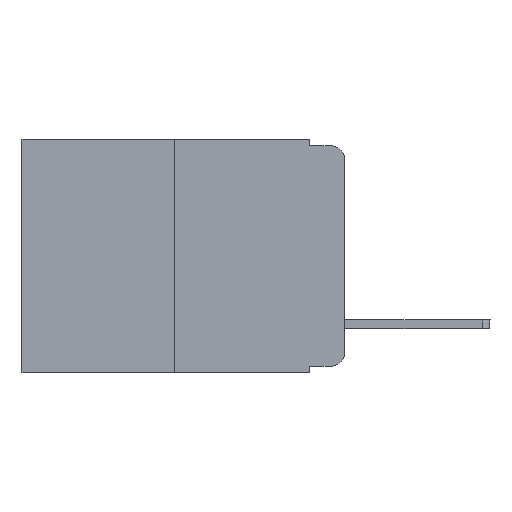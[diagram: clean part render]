
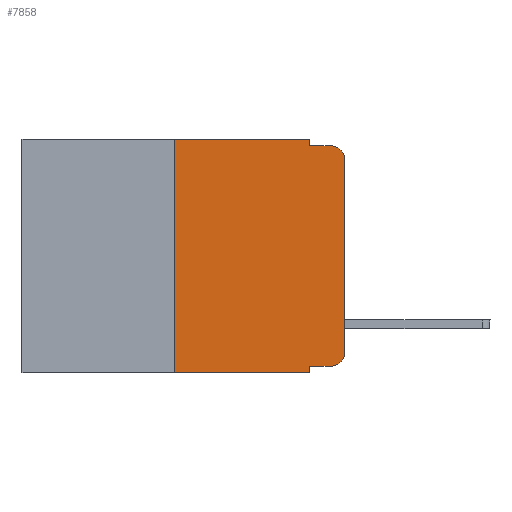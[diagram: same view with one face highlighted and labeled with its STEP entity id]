
A CAD part, left-side view. The second image highlights one B-rep face of the part: STEP entity #7858.
In plain terms, the highlighted planar face has unit normal (-1, 0, 0).
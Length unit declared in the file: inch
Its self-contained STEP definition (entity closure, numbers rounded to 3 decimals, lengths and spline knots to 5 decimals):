
#303 = DIRECTION ( 'NONE',  ( 0., 0., -1. ) ) ;
#461 = CARTESIAN_POINT ( 'NONE',  ( 0., 0., -0.03 ) ) ;
#546 = DIRECTION ( 'NONE',  ( 0., -1., 0. ) ) ;
#664 = VECTOR ( 'NONE', #1837, 39.37008 ) ;
#684 = ORIENTED_EDGE ( 'NONE', *, *, #11187, .F. ) ;
#804 = ORIENTED_EDGE ( 'NONE', *, *, #11009, .F. ) ;
#863 = LINE ( 'NONE', #10793, #5171 ) ;
#924 = DIRECTION ( 'NONE',  ( 0., 0., -1. ) ) ;
#939 = CARTESIAN_POINT ( 'NONE',  ( 0., 0.473, -0.343 ) ) ;
#1237 = DIRECTION ( 'NONE',  ( 0., 0., -1. ) ) ;
#1802 = EDGE_CURVE ( 'NONE', #3468, #7942, #8246, .T. ) ;
#1824 = EDGE_CURVE ( 'NONE', #2401, #6119, #2225, .T. ) ;
#1837 = DIRECTION ( 'NONE',  ( 0., 0., -1. ) ) ;
#1941 = CARTESIAN_POINT ( 'NONE',  ( 0., 0.051, -0.01 ) ) ;
#1979 = VERTEX_POINT ( 'NONE', #6339 ) ;
#2007 = LINE ( 'NONE', #2062, #664 ) ;
#2062 = CARTESIAN_POINT ( 'NONE',  ( 0., 0.051, 0. ) ) ;
#2225 = LINE ( 'NONE', #6740, #9524 ) ;
#2401 = VERTEX_POINT ( 'NONE', #6045 ) ;
#2422 = CIRCLE ( 'NONE', #5268, 0.02 ) ;
#2423 = CARTESIAN_POINT ( 'NONE',  ( 0., 0.25, 0. ) ) ;
#2510 = DIRECTION ( 'NONE',  ( 0., -1., 0. ) ) ;
#2691 = ORIENTED_EDGE ( 'NONE', *, *, #11064, .T. ) ;
#2708 = CARTESIAN_POINT ( 'NONE',  ( 0., 0.02, -0.03 ) ) ;
#2950 = VERTEX_POINT ( 'NONE', #461 ) ;
#3108 = ORIENTED_EDGE ( 'NONE', *, *, #4291, .T. ) ;
#3150 = EDGE_CURVE ( 'NONE', #2401, #1979, #2007, .T. ) ;
#3179 = DIRECTION ( 'NONE',  ( 0., -1., 0. ) ) ;
#3212 = ORIENTED_EDGE ( 'NONE', *, *, #4477, .T. ) ;
#3214 = FACE_OUTER_BOUND ( 'NONE', #11480, .T. ) ;
#3459 = CARTESIAN_POINT ( 'NONE',  ( 0., 0.25, -0.343 ) ) ;
#3468 = VERTEX_POINT ( 'NONE', #8184 ) ;
#3621 = DIRECTION ( 'NONE',  ( 0., 0., 1. ) ) ;
#3765 = AXIS2_PLACEMENT_3D ( 'NONE', #8465, #7506, #303 ) ;
#4149 = VERTEX_POINT ( 'NONE', #2423 ) ;
#4291 = EDGE_CURVE ( 'NONE', #2950, #7942, #2422, .T. ) ;
#4418 = LINE ( 'NONE', #939, #5251 ) ;
#4477 = EDGE_CURVE ( 'NONE', #6119, #10706, #10963, .T. ) ;
#4743 = CARTESIAN_POINT ( 'NONE',  ( 0., 0.051, 0. ) ) ;
#5020 = EDGE_CURVE ( 'NONE', #7541, #1979, #4418, .T. ) ;
#5062 = ORIENTED_EDGE ( 'NONE', *, *, #5020, .T. ) ;
#5171 = VECTOR ( 'NONE', #7955, 39.37008 ) ;
#5251 = VECTOR ( 'NONE', #2510, 39.37008 ) ;
#5268 = AXIS2_PLACEMENT_3D ( 'NONE', #2708, #10848, #8948 ) ;
#5687 = ORIENTED_EDGE ( 'NONE', *, *, #1824, .T. ) ;
#5882 = ORIENTED_EDGE ( 'NONE', *, *, #6718, .F. ) ;
#5905 = VERTEX_POINT ( 'NONE', #4743 ) ;
#6045 = CARTESIAN_POINT ( 'NONE',  ( 0., 0.051, -0.333 ) ) ;
#6119 = VERTEX_POINT ( 'NONE', #10836 ) ;
#6256 = VECTOR ( 'NONE', #924, 39.37008 ) ;
#6339 = CARTESIAN_POINT ( 'NONE',  ( 0., 0.051, -0.343 ) ) ;
#6452 = VECTOR ( 'NONE', #3621, 39.37008 ) ;
#6718 = EDGE_CURVE ( 'NONE', #4149, #5905, #863, .T. ) ;
#6740 = CARTESIAN_POINT ( 'NONE',  ( 0., 0.051, -0.333 ) ) ;
#6942 = LINE ( 'NONE', #8027, #11109 ) ;
#7023 = ORIENTED_EDGE ( 'NONE', *, *, #1802, .F. ) ;
#7179 = CARTESIAN_POINT ( 'NONE',  ( 0., 0., 0. ) ) ;
#7448 = ORIENTED_EDGE ( 'NONE', *, *, #3150, .F. ) ;
#7506 = DIRECTION ( 'NONE',  ( -1., 0., 0. ) ) ;
#7541 = VERTEX_POINT ( 'NONE', #3459 ) ;
#7779 = DIRECTION ( 'NONE',  ( 0., 0., 1. ) ) ;
#7858 = ADVANCED_FACE ( 'NONE', ( #3214 ), #9565, .F. ) ;
#7942 = VERTEX_POINT ( 'NONE', #8036 ) ;
#7955 = DIRECTION ( 'NONE',  ( 0., -1., 0. ) ) ;
#8027 = CARTESIAN_POINT ( 'NONE',  ( 0., 0.25, 0. ) ) ;
#8036 = CARTESIAN_POINT ( 'NONE',  ( 0., 0.02, -0.01 ) ) ;
#8184 = CARTESIAN_POINT ( 'NONE',  ( 0., 0.051, -0.01 ) ) ;
#8208 = CARTESIAN_POINT ( 'NONE',  ( 0., 0., -0.313 ) ) ;
#8246 = LINE ( 'NONE', #1941, #11054 ) ;
#8465 = CARTESIAN_POINT ( 'NONE',  ( 0., 0.02, -0.313 ) ) ;
#8936 = AXIS2_PLACEMENT_3D ( 'NONE', #9394, #10456, #1237 ) ;
#8948 = DIRECTION ( 'NONE',  ( 0., 0., -1. ) ) ;
#9083 = LINE ( 'NONE', #10928, #6256 ) ;
#9394 = CARTESIAN_POINT ( 'NONE',  ( 0., 0.473, 0. ) ) ;
#9524 = VECTOR ( 'NONE', #3179, 39.37008 ) ;
#9565 = PLANE ( 'NONE',  #8936 ) ;
#10456 = DIRECTION ( 'NONE',  ( 1., 0., 0. ) ) ;
#10706 = VERTEX_POINT ( 'NONE', #8208 ) ;
#10793 = CARTESIAN_POINT ( 'NONE',  ( 0., 0.473, 0. ) ) ;
#10836 = CARTESIAN_POINT ( 'NONE',  ( 0., 0.02, -0.333 ) ) ;
#10848 = DIRECTION ( 'NONE',  ( -1., 0., 0. ) ) ;
#10928 = CARTESIAN_POINT ( 'NONE',  ( 0., 0.051, 0. ) ) ;
#10963 = CIRCLE ( 'NONE', #3765, 0.02 ) ;
#11009 = EDGE_CURVE ( 'NONE', #7541, #4149, #6942, .T. ) ;
#11054 = VECTOR ( 'NONE', #546, 39.37008 ) ;
#11064 = EDGE_CURVE ( 'NONE', #10706, #2950, #11697, .T. ) ;
#11109 = VECTOR ( 'NONE', #7779, 39.37008 ) ;
#11187 = EDGE_CURVE ( 'NONE', #5905, #3468, #9083, .T. ) ;
#11480 = EDGE_LOOP ( 'NONE', ( #2691, #3108, #7023, #684, #5882, #804, #5062, #7448, #5687, #3212 ) ) ;
#11697 = LINE ( 'NONE', #7179, #6452 ) ;
